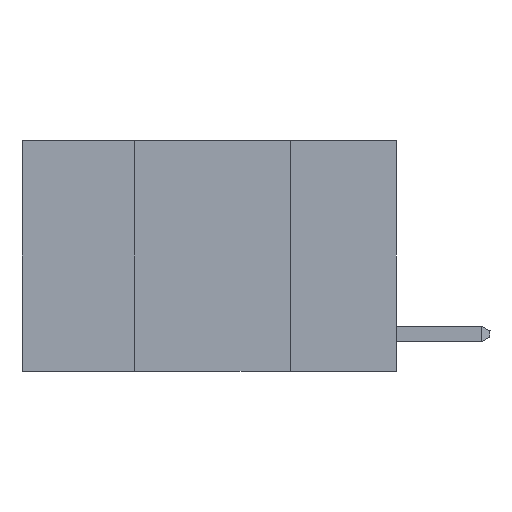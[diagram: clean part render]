
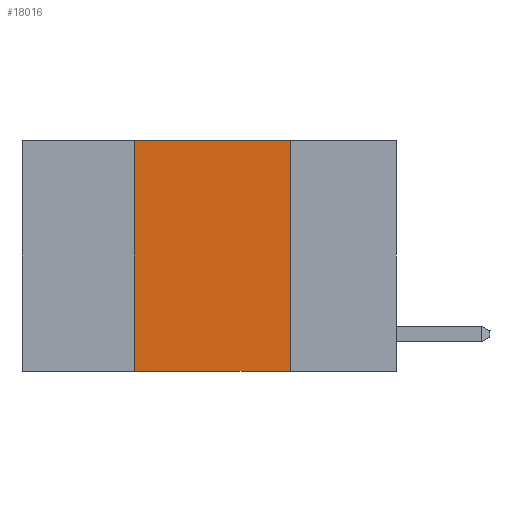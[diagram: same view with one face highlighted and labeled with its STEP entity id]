
A CAD part, left-side view. The second image highlights one B-rep face of the part: STEP entity #18016.
In plain terms, the highlighted planar face has unit normal (-1, 0, 0).
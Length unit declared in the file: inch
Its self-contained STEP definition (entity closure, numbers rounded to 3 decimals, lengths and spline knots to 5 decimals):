
#206 = DIRECTION ( 'NONE',  ( 0., 0., -1. ) ) ;
#227 = CARTESIAN_POINT ( 'NONE',  ( 0., 0.17, 0. ) ) ;
#1310 = EDGE_CURVE ( 'NONE', #5947, #3134, #20155, .T. ) ;
#2177 = CARTESIAN_POINT ( 'NONE',  ( 0., 0.17, -0.37 ) ) ;
#2581 = VERTEX_POINT ( 'NONE', #4663 ) ;
#3122 = VECTOR ( 'NONE', #23021, 39.37008 ) ;
#3134 = VERTEX_POINT ( 'NONE', #2177 ) ;
#3347 = AXIS2_PLACEMENT_3D ( 'NONE', #17407, #21129, #10038 ) ;
#3687 = LINE ( 'NONE', #17485, #3122 ) ;
#4056 = VECTOR ( 'NONE', #5545, 39.37008 ) ;
#4663 = CARTESIAN_POINT ( 'NONE',  ( 0., 0.42, 0. ) ) ;
#5488 = CARTESIAN_POINT ( 'NONE',  ( 0., 0.17, 0. ) ) ;
#5545 = DIRECTION ( 'NONE',  ( 0., 0., 1. ) ) ;
#5689 = CARTESIAN_POINT ( 'NONE',  ( 0., 0.42, -0.37 ) ) ;
#5947 = VERTEX_POINT ( 'NONE', #5488 ) ;
#6523 = EDGE_CURVE ( 'NONE', #18484, #2581, #23608, .T. ) ;
#6552 = LINE ( 'NONE', #9376, #10835 ) ;
#7468 = DIRECTION ( 'NONE',  ( 0., -1., 0. ) ) ;
#8117 = PLANE ( 'NONE',  #3347 ) ;
#9376 = CARTESIAN_POINT ( 'NONE',  ( 0., 0.6, -0.37 ) ) ;
#10038 = DIRECTION ( 'NONE',  ( 0., 0., -1. ) ) ;
#10835 = VECTOR ( 'NONE', #7468, 39.37008 ) ;
#12898 = EDGE_CURVE ( 'NONE', #2581, #5947, #3687, .T. ) ;
#13150 = EDGE_CURVE ( 'NONE', #18484, #3134, #6552, .T. ) ;
#17407 = CARTESIAN_POINT ( 'NONE',  ( 0., 0.6, 0. ) ) ;
#17485 = CARTESIAN_POINT ( 'NONE',  ( 0., 0.6, 0. ) ) ;
#18016 = ADVANCED_FACE ( 'NONE', ( #18941 ), #8117, .F. ) ;
#18217 = EDGE_LOOP ( 'NONE', ( #19231, #18690, #18853, #19474 ) ) ;
#18484 = VERTEX_POINT ( 'NONE', #5689 ) ;
#18690 = ORIENTED_EDGE ( 'NONE', *, *, #12898, .F. ) ;
#18853 = ORIENTED_EDGE ( 'NONE', *, *, #6523, .F. ) ;
#18941 = FACE_OUTER_BOUND ( 'NONE', #18217, .T. ) ;
#19004 = VECTOR ( 'NONE', #206, 39.37008 ) ;
#19231 = ORIENTED_EDGE ( 'NONE', *, *, #1310, .F. ) ;
#19474 = ORIENTED_EDGE ( 'NONE', *, *, #13150, .T. ) ;
#20155 = LINE ( 'NONE', #227, #19004 ) ;
#20326 = CARTESIAN_POINT ( 'NONE',  ( 0., 0.42, 0. ) ) ;
#21129 = DIRECTION ( 'NONE',  ( 1., 0., 0. ) ) ;
#23021 = DIRECTION ( 'NONE',  ( 0., -1., 0. ) ) ;
#23608 = LINE ( 'NONE', #20326, #4056 ) ;
